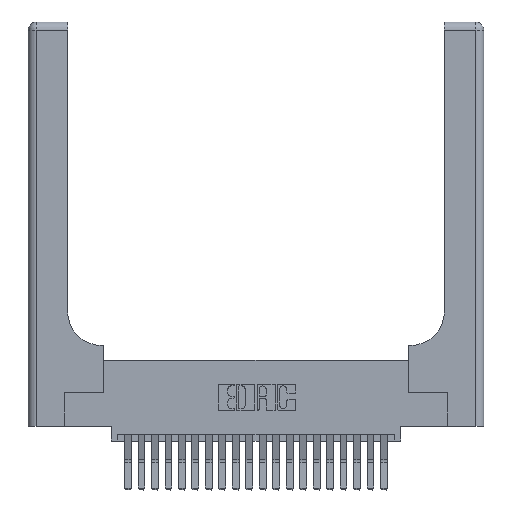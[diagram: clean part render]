
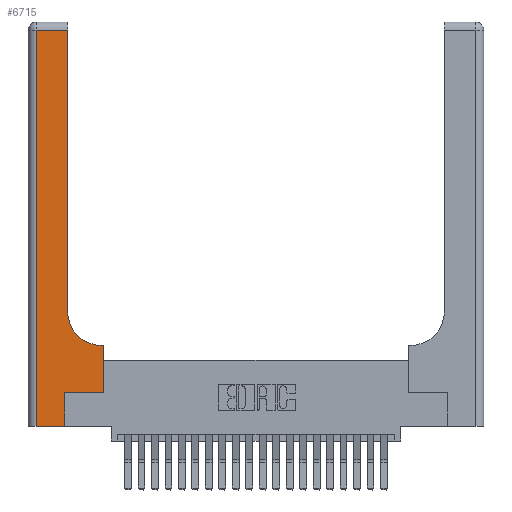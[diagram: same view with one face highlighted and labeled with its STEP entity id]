
A CAD part, top view. The second image highlights one B-rep face of the part: STEP entity #6715.
In plain terms, the highlighted planar face has unit normal (0, 0, 1).
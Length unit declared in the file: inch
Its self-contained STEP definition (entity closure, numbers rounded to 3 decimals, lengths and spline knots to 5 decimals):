
#58 = EDGE_LOOP ( 'NONE', ( #10759, #7476, #9617, #14270, #22605, #8519, #17599, #17993, #14121 ) ) ;
#343 = VECTOR ( 'NONE', #5544, 39.37008 ) ;
#413 = CARTESIAN_POINT ( 'NONE',  ( 0.2915, 2.94, 0.37 ) ) ;
#1649 = VECTOR ( 'NONE', #15802, 39.37008 ) ;
#1681 = EDGE_CURVE ( 'NONE', #10204, #21914, #4040, .T. ) ;
#1862 = CARTESIAN_POINT ( 'NONE',  ( 0.5585, 0.25, 0.37 ) ) ;
#3033 = VERTEX_POINT ( 'NONE', #14329 ) ;
#3377 = CARTESIAN_POINT ( 'NONE',  ( 0., 3., 0.37 ) ) ;
#3779 = DIRECTION ( 'NONE',  ( 0., 1., 0. ) ) ;
#3897 = EDGE_CURVE ( 'NONE', #17750, #21455, #6013, .T. ) ;
#3901 = VECTOR ( 'NONE', #23120, 39.37008 ) ;
#4040 = LINE ( 'NONE', #19490, #1649 ) ;
#5474 = VERTEX_POINT ( 'NONE', #18308 ) ;
#5544 = DIRECTION ( 'NONE',  ( -1., 0., 0. ) ) ;
#5960 = VECTOR ( 'NONE', #3779, 39.37008 ) ;
#5998 = LINE ( 'NONE', #8873, #10993 ) ;
#6013 = LINE ( 'NONE', #18491, #343 ) ;
#6198 = AXIS2_PLACEMENT_3D ( 'NONE', #7924, #20840, #9827 ) ;
#6715 = ADVANCED_FACE ( 'NONE', ( #7334 ), #14533, .F. ) ;
#7334 = FACE_OUTER_BOUND ( 'NONE', #58, .T. ) ;
#7476 = ORIENTED_EDGE ( 'NONE', *, *, #3897, .T. ) ;
#7639 = AXIS2_PLACEMENT_3D ( 'NONE', #3377, #20080, #9049 ) ;
#7786 = CARTESIAN_POINT ( 'NONE',  ( 0.2915, 3., 0.37 ) ) ;
#7924 = CARTESIAN_POINT ( 'NONE',  ( 0.5415, 0.85, 0.37 ) ) ;
#8386 = LINE ( 'NONE', #7786, #13339 ) ;
#8519 = ORIENTED_EDGE ( 'NONE', *, *, #11291, .T. ) ;
#8782 = DIRECTION ( 'NONE',  ( 0., -1., 0. ) ) ;
#8873 = CARTESIAN_POINT ( 'NONE',  ( 0.269, 0.25, 0.37 ) ) ;
#8882 = LINE ( 'NONE', #21238, #3901 ) ;
#9049 = DIRECTION ( 'NONE',  ( -1., 0., 0. ) ) ;
#9096 = CARTESIAN_POINT ( 'NONE',  ( 0.5415, 0.6, 0.37 ) ) ;
#9214 = CARTESIAN_POINT ( 'NONE',  ( 0.269, 0.25, 0.37 ) ) ;
#9617 = ORIENTED_EDGE ( 'NONE', *, *, #19469, .T. ) ;
#9625 = CARTESIAN_POINT ( 'NONE',  ( 0.2915, 0.6, 0.37 ) ) ;
#9827 = DIRECTION ( 'NONE',  ( 1., 0., 0. ) ) ;
#10204 = VERTEX_POINT ( 'NONE', #24083 ) ;
#10759 = ORIENTED_EDGE ( 'NONE', *, *, #23743, .T. ) ;
#10993 = VECTOR ( 'NONE', #21746, 39.37008 ) ;
#11291 = EDGE_CURVE ( 'NONE', #21914, #17094, #5998, .T. ) ;
#12125 = LINE ( 'NONE', #1862, #5960 ) ;
#12818 = CARTESIAN_POINT ( 'NONE',  ( 0.2915, 0.85, 0.37 ) ) ;
#13269 = LINE ( 'NONE', #23373, #18147 ) ;
#13339 = VECTOR ( 'NONE', #18902, 39.37008 ) ;
#13485 = EDGE_CURVE ( 'NONE', #16202, #21278, #22492, .T. ) ;
#14121 = ORIENTED_EDGE ( 'NONE', *, *, #13485, .T. ) ;
#14270 = ORIENTED_EDGE ( 'NONE', *, *, #15354, .T. ) ;
#14329 = CARTESIAN_POINT ( 'NONE',  ( 0.5585, 0.6, 0.37 ) ) ;
#14533 = PLANE ( 'NONE',  #7639 ) ;
#15354 = EDGE_CURVE ( 'NONE', #5474, #10204, #8882, .T. ) ;
#15802 = DIRECTION ( 'NONE',  ( 0., 1., 0. ) ) ;
#16202 = VERTEX_POINT ( 'NONE', #9096 ) ;
#17094 = VERTEX_POINT ( 'NONE', #20973 ) ;
#17599 = ORIENTED_EDGE ( 'NONE', *, *, #19596, .T. ) ;
#17750 = VERTEX_POINT ( 'NONE', #413 ) ;
#17993 = ORIENTED_EDGE ( 'NONE', *, *, #20741, .T. ) ;
#18147 = VECTOR ( 'NONE', #8782, 39.37008 ) ;
#18308 = CARTESIAN_POINT ( 'NONE',  ( 0.06, 0., 0.37 ) ) ;
#18491 = CARTESIAN_POINT ( 'NONE',  ( 0., 2.94, 0.37 ) ) ;
#18902 = DIRECTION ( 'NONE',  ( 0., 1., 0. ) ) ;
#19469 = EDGE_CURVE ( 'NONE', #21455, #5474, #13269, .T. ) ;
#19490 = CARTESIAN_POINT ( 'NONE',  ( 0.269, 0., 0.37 ) ) ;
#19596 = EDGE_CURVE ( 'NONE', #17094, #3033, #12125, .T. ) ;
#20080 = DIRECTION ( 'NONE',  ( 0., 0., -1. ) ) ;
#20741 = EDGE_CURVE ( 'NONE', #3033, #16202, #24047, .T. ) ;
#20840 = DIRECTION ( 'NONE',  ( 0., 0., -1. ) ) ;
#20973 = CARTESIAN_POINT ( 'NONE',  ( 0.5585, 0.25, 0.37 ) ) ;
#21238 = CARTESIAN_POINT ( 'NONE',  ( 0., 0., 0.37 ) ) ;
#21278 = VERTEX_POINT ( 'NONE', #12818 ) ;
#21455 = VERTEX_POINT ( 'NONE', #22577 ) ;
#21746 = DIRECTION ( 'NONE',  ( 1., 0., 0. ) ) ;
#21914 = VERTEX_POINT ( 'NONE', #9214 ) ;
#22456 = DIRECTION ( 'NONE',  ( -1., 0., 0. ) ) ;
#22492 = CIRCLE ( 'NONE', #6198, 0.25 ) ;
#22577 = CARTESIAN_POINT ( 'NONE',  ( 0.06, 2.94, 0.37 ) ) ;
#22605 = ORIENTED_EDGE ( 'NONE', *, *, #1681, .T. ) ;
#23120 = DIRECTION ( 'NONE',  ( 1., 0., 0. ) ) ;
#23373 = CARTESIAN_POINT ( 'NONE',  ( 0.06, 3., 0.37 ) ) ;
#23459 = VECTOR ( 'NONE', #22456, 39.37008 ) ;
#23743 = EDGE_CURVE ( 'NONE', #21278, #17750, #8386, .T. ) ;
#24047 = LINE ( 'NONE', #9625, #23459 ) ;
#24083 = CARTESIAN_POINT ( 'NONE',  ( 0.269, 0., 0.37 ) ) ;
